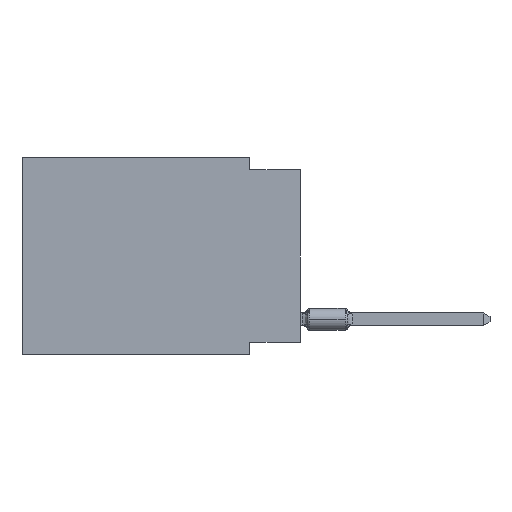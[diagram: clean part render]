
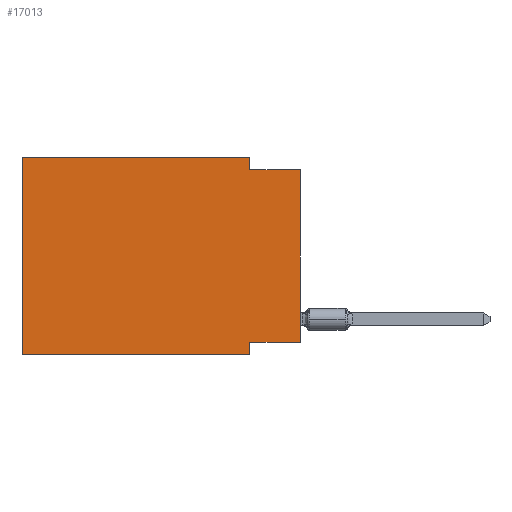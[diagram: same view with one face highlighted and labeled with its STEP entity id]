
A CAD part, left-side view. The second image highlights one B-rep face of the part: STEP entity #17013.
In plain terms, the highlighted planar face has unit normal (-1, 0, 0).
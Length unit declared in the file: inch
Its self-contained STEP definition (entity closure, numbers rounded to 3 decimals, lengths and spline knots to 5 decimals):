
#131 = DIRECTION ( 'NONE',  ( 0., 0., -1. ) ) ;
#148 = LINE ( 'NONE', #1620, #5574 ) ;
#336 = VECTOR ( 'NONE', #131, 39.37008 ) ;
#451 = ORIENTED_EDGE ( 'NONE', *, *, #17263, .F. ) ;
#704 = EDGE_CURVE ( 'NONE', #4197, #8761, #8256, .T. ) ;
#1002 = EDGE_CURVE ( 'NONE', #7335, #8761, #1231, .T. ) ;
#1231 = LINE ( 'NONE', #4180, #1430 ) ;
#1344 = VERTEX_POINT ( 'NONE', #16906 ) ;
#1430 = VECTOR ( 'NONE', #6849, 39.37008 ) ;
#1620 = CARTESIAN_POINT ( 'NONE',  ( 0., 0.55, 0. ) ) ;
#1653 = LINE ( 'NONE', #8666, #16929 ) ;
#2128 = CARTESIAN_POINT ( 'NONE',  ( 0., 0., -0.365 ) ) ;
#2552 = ORIENTED_EDGE ( 'NONE', *, *, #3105, .F. ) ;
#2612 = EDGE_CURVE ( 'NONE', #1344, #13264, #10263, .T. ) ;
#3105 = EDGE_CURVE ( 'NONE', #1344, #4197, #13752, .T. ) ;
#3551 = CARTESIAN_POINT ( 'NONE',  ( 0., 0., -0.025 ) ) ;
#3800 = CARTESIAN_POINT ( 'NONE',  ( 0., 0.1, 0. ) ) ;
#4180 = CARTESIAN_POINT ( 'NONE',  ( 0., 0.55, -0.39 ) ) ;
#4197 = VERTEX_POINT ( 'NONE', #5548 ) ;
#4722 = VECTOR ( 'NONE', #15913, 39.37008 ) ;
#5064 = EDGE_CURVE ( 'NONE', #15264, #7296, #148, .T. ) ;
#5548 = CARTESIAN_POINT ( 'NONE',  ( 0., 0.1, -0.365 ) ) ;
#5574 = VECTOR ( 'NONE', #5954, 39.37008 ) ;
#5711 = VECTOR ( 'NONE', #9424, 39.37008 ) ;
#5954 = DIRECTION ( 'NONE',  ( 0., -1., 0. ) ) ;
#6336 = LINE ( 'NONE', #7809, #12566 ) ;
#6382 = CARTESIAN_POINT ( 'NONE',  ( 0., 0.55, 0. ) ) ;
#6518 = DIRECTION ( 'NONE',  ( 0., 0., 1. ) ) ;
#6676 = VECTOR ( 'NONE', #11911, 39.37008 ) ;
#6849 = DIRECTION ( 'NONE',  ( 0., -1., 0. ) ) ;
#7069 = ORIENTED_EDGE ( 'NONE', *, *, #9998, .F. ) ;
#7296 = VERTEX_POINT ( 'NONE', #14751 ) ;
#7335 = VERTEX_POINT ( 'NONE', #16322 ) ;
#7809 = CARTESIAN_POINT ( 'NONE',  ( 0., 0.55, 0. ) ) ;
#8256 = LINE ( 'NONE', #13990, #336 ) ;
#8289 = CARTESIAN_POINT ( 'NONE',  ( 0., 0.1, -0.025 ) ) ;
#8641 = ORIENTED_EDGE ( 'NONE', *, *, #2612, .T. ) ;
#8666 = CARTESIAN_POINT ( 'NONE',  ( 0., 0., -0.025 ) ) ;
#8761 = VERTEX_POINT ( 'NONE', #11998 ) ;
#8964 = DIRECTION ( 'NONE',  ( 1., 0., 0. ) ) ;
#9424 = DIRECTION ( 'NONE',  ( 0., 0., -1. ) ) ;
#9998 = EDGE_CURVE ( 'NONE', #7335, #15264, #6336, .T. ) ;
#10263 = LINE ( 'NONE', #17494, #4722 ) ;
#11121 = EDGE_CURVE ( 'NONE', #15952, #13264, #1653, .T. ) ;
#11532 = DIRECTION ( 'NONE',  ( 0., -1., 0. ) ) ;
#11647 = DIRECTION ( 'NONE',  ( 0., 0., -1. ) ) ;
#11911 = DIRECTION ( 'NONE',  ( 0., 1., 0. ) ) ;
#11998 = CARTESIAN_POINT ( 'NONE',  ( 0., 0.1, -0.39 ) ) ;
#12566 = VECTOR ( 'NONE', #6518, 39.37008 ) ;
#13264 = VERTEX_POINT ( 'NONE', #3551 ) ;
#13752 = LINE ( 'NONE', #2128, #6676 ) ;
#13990 = CARTESIAN_POINT ( 'NONE',  ( 0., 0.1, -0.39 ) ) ;
#14428 = FACE_OUTER_BOUND ( 'NONE', #15760, .T. ) ;
#14751 = CARTESIAN_POINT ( 'NONE',  ( 0., 0.1, 0. ) ) ;
#15177 = ORIENTED_EDGE ( 'NONE', *, *, #5064, .F. ) ;
#15264 = VERTEX_POINT ( 'NONE', #16410 ) ;
#15670 = ORIENTED_EDGE ( 'NONE', *, *, #1002, .T. ) ;
#15760 = EDGE_LOOP ( 'NONE', ( #8641, #17238, #451, #15177, #7069, #15670, #18163, #2552 ) ) ;
#15913 = DIRECTION ( 'NONE',  ( 0., 0., 1. ) ) ;
#15952 = VERTEX_POINT ( 'NONE', #8289 ) ;
#16099 = PLANE ( 'NONE',  #17812 ) ;
#16322 = CARTESIAN_POINT ( 'NONE',  ( 0., 0.55, -0.39 ) ) ;
#16410 = CARTESIAN_POINT ( 'NONE',  ( 0., 0.55, 0. ) ) ;
#16465 = LINE ( 'NONE', #3800, #5711 ) ;
#16906 = CARTESIAN_POINT ( 'NONE',  ( 0., 0., -0.365 ) ) ;
#16929 = VECTOR ( 'NONE', #11532, 39.37008 ) ;
#17013 = ADVANCED_FACE ( 'NONE', ( #14428 ), #16099, .F. ) ;
#17238 = ORIENTED_EDGE ( 'NONE', *, *, #11121, .F. ) ;
#17263 = EDGE_CURVE ( 'NONE', #7296, #15952, #16465, .T. ) ;
#17494 = CARTESIAN_POINT ( 'NONE',  ( 0., 0., 0. ) ) ;
#17812 = AXIS2_PLACEMENT_3D ( 'NONE', #6382, #8964, #11647 ) ;
#18163 = ORIENTED_EDGE ( 'NONE', *, *, #704, .F. ) ;
